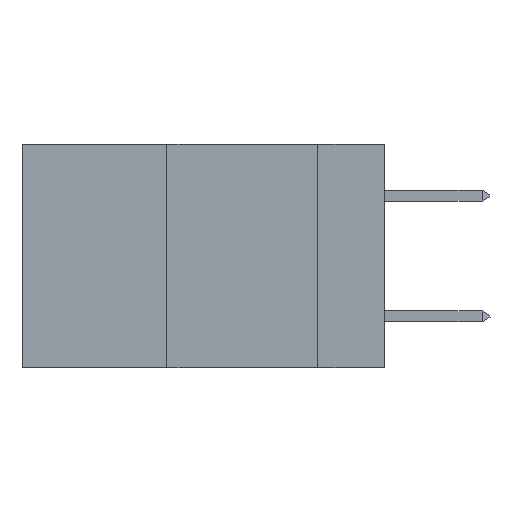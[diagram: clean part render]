
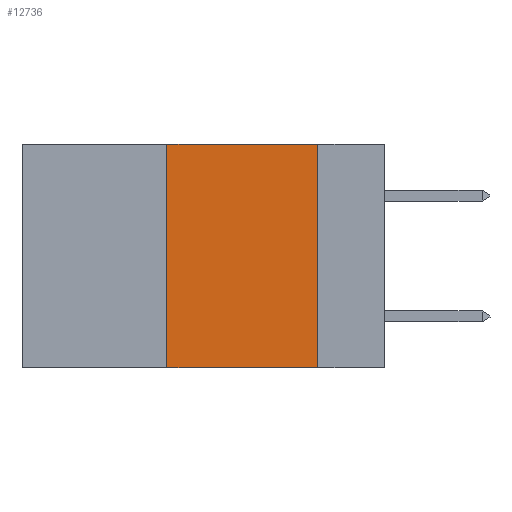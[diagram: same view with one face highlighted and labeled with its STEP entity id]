
A CAD part, left-side view. The second image highlights one B-rep face of the part: STEP entity #12736.
In plain terms, the highlighted planar face has unit normal (-1, 0, 0).
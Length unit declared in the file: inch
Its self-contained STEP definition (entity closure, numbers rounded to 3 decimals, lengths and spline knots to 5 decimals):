
#226 = DIRECTION ( 'NONE',  ( 0., 0., -1. ) ) ;
#633 = DIRECTION ( 'NONE',  ( 0., -1., 0. ) ) ;
#803 = ORIENTED_EDGE ( 'NONE', *, *, #17086, .F. ) ;
#1872 = ORIENTED_EDGE ( 'NONE', *, *, #8908, .F. ) ;
#2449 = VECTOR ( 'NONE', #16662, 39.37008 ) ;
#3918 = LINE ( 'NONE', #14417, #19276 ) ;
#4340 = VECTOR ( 'NONE', #5257, 39.37008 ) ;
#5257 = DIRECTION ( 'NONE',  ( 0., 0., 1. ) ) ;
#5283 = CARTESIAN_POINT ( 'NONE',  ( 0., 0.6, 0. ) ) ;
#5890 = EDGE_CURVE ( 'NONE', #8620, #16705, #10412, .T. ) ;
#5895 = FACE_OUTER_BOUND ( 'NONE', #6176, .T. ) ;
#6176 = EDGE_LOOP ( 'NONE', ( #18535, #803, #1872, #6949 ) ) ;
#6368 = CARTESIAN_POINT ( 'NONE',  ( 0., 0.36, 0. ) ) ;
#6856 = DIRECTION ( 'NONE',  ( 0., 0., -1. ) ) ;
#6887 = EDGE_CURVE ( 'NONE', #12774, #16705, #3918, .T. ) ;
#6919 = CARTESIAN_POINT ( 'NONE',  ( 0., 0.36, -0.37 ) ) ;
#6949 = ORIENTED_EDGE ( 'NONE', *, *, #6887, .T. ) ;
#7338 = VERTEX_POINT ( 'NONE', #6368 ) ;
#8382 = LINE ( 'NONE', #14234, #4340 ) ;
#8620 = VERTEX_POINT ( 'NONE', #15149 ) ;
#8908 = EDGE_CURVE ( 'NONE', #12774, #7338, #8382, .T. ) ;
#10066 = LINE ( 'NONE', #13879, #2449 ) ;
#10163 = CARTESIAN_POINT ( 'NONE',  ( 0., 0.11, -0.37 ) ) ;
#10412 = LINE ( 'NONE', #15534, #17760 ) ;
#12736 = ADVANCED_FACE ( 'NONE', ( #5895 ), #12905, .F. ) ;
#12774 = VERTEX_POINT ( 'NONE', #6919 ) ;
#12905 = PLANE ( 'NONE',  #15963 ) ;
#13879 = CARTESIAN_POINT ( 'NONE',  ( 0., 0.6, 0. ) ) ;
#14234 = CARTESIAN_POINT ( 'NONE',  ( 0., 0.36, 0. ) ) ;
#14417 = CARTESIAN_POINT ( 'NONE',  ( 0., 0.6, -0.37 ) ) ;
#15149 = CARTESIAN_POINT ( 'NONE',  ( 0., 0.11, 0. ) ) ;
#15534 = CARTESIAN_POINT ( 'NONE',  ( 0., 0.11, 0. ) ) ;
#15784 = DIRECTION ( 'NONE',  ( 1., 0., 0. ) ) ;
#15963 = AXIS2_PLACEMENT_3D ( 'NONE', #5283, #15784, #6856 ) ;
#16662 = DIRECTION ( 'NONE',  ( 0., -1., 0. ) ) ;
#16705 = VERTEX_POINT ( 'NONE', #10163 ) ;
#17086 = EDGE_CURVE ( 'NONE', #7338, #8620, #10066, .T. ) ;
#17760 = VECTOR ( 'NONE', #226, 39.37008 ) ;
#18535 = ORIENTED_EDGE ( 'NONE', *, *, #5890, .F. ) ;
#19276 = VECTOR ( 'NONE', #633, 39.37008 ) ;
